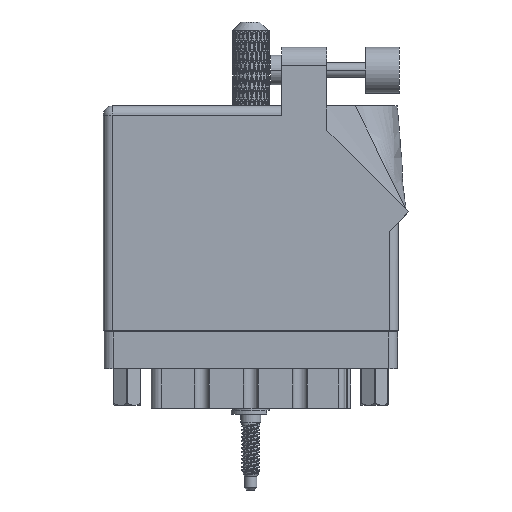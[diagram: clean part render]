
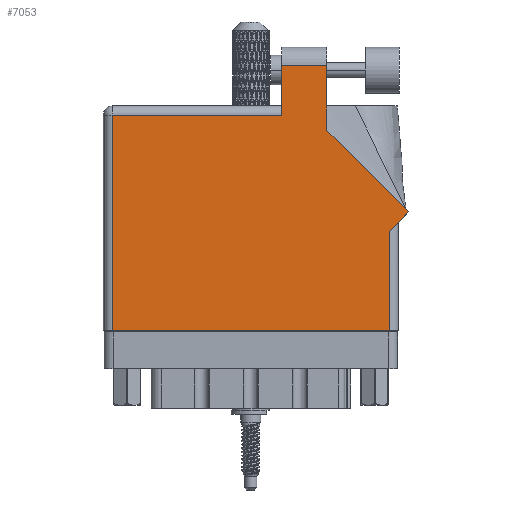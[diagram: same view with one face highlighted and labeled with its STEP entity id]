
A CAD part, front view. The second image highlights one B-rep face of the part: STEP entity #7053.
In plain terms, the highlighted face is planar.
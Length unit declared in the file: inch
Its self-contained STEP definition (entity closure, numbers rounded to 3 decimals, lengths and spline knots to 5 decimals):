
#5122 = VECTOR ( 'NONE', #75772, 39.37008 ) ;
#7053 = ADVANCED_FACE ( 'NONE', ( #70949 ), #7732, .F. ) ;
#7732 = PLANE ( 'NONE',  #76539 ) ;
#9348 = VERTEX_POINT ( 'NONE', #70946 ) ;
#9827 = EDGE_CURVE ( 'NONE', #87743, #76455, #40275, .T. ) ;
#10500 = VERTEX_POINT ( 'NONE', #101364 ) ;
#10588 = LINE ( 'NONE', #63871, #114702 ) ;
#10964 = DIRECTION ( 'NONE',  ( -0.707, 0.707, 0. ) ) ;
#11872 = CARTESIAN_POINT ( 'NONE',  ( 0., 0., 0. ) ) ;
#19192 = CARTESIAN_POINT ( 'NONE',  ( 2.08071, 0.80771, 0. ) ) ;
#19489 = LINE ( 'NONE', #11872, #102658 ) ;
#20319 = LINE ( 'NONE', #19192, #86855 ) ;
#21005 = EDGE_CURVE ( 'NONE', #69353, #87743, #53321, .T. ) ;
#24170 = DIRECTION ( 'NONE',  ( 0., 1., 0. ) ) ;
#26966 = CARTESIAN_POINT ( 'NONE',  ( 1.217, 1.53, 0. ) ) ;
#28724 = CARTESIAN_POINT ( 'NONE',  ( 0.062, 0., 0. ) ) ;
#29617 = CARTESIAN_POINT ( 'NONE',  ( 1.524, 1.36442, 0. ) ) ;
#31283 = ORIENTED_EDGE ( 'NONE', *, *, #49875, .T. ) ;
#36692 = CARTESIAN_POINT ( 'NONE',  ( 1.948, 0.675, 0. ) ) ;
#36913 = EDGE_CURVE ( 'NONE', #74993, #54973, #49385, .T. ) ;
#40275 = LINE ( 'NONE', #84242, #65567 ) ;
#45832 = DIRECTION ( 'NONE',  ( 1., 0., 0. ) ) ;
#45952 = CARTESIAN_POINT ( 'NONE',  ( 1.217, 1.805, 0. ) ) ;
#46294 = DIRECTION ( 'NONE',  ( -1., 0., 0. ) ) ;
#48882 = ORIENTED_EDGE ( 'NONE', *, *, #9827, .T. ) ;
#49385 = LINE ( 'NONE', #74615, #5122 ) ;
#49875 = EDGE_CURVE ( 'NONE', #76455, #114369, #55099, .T. ) ;
#52419 = VERTEX_POINT ( 'NONE', #78527 ) ;
#53061 = EDGE_CURVE ( 'NONE', #114369, #52419, #19489, .T. ) ;
#53321 = LINE ( 'NONE', #26966, #95538 ) ;
#53946 = DIRECTION ( 'NONE',  ( 0., 0., -1. ) ) ;
#54632 = ORIENTED_EDGE ( 'NONE', *, *, #82011, .T. ) ;
#54973 = VERTEX_POINT ( 'NONE', #89407 ) ;
#55099 = LINE ( 'NONE', #28724, #55949 ) ;
#55949 = VECTOR ( 'NONE', #88098, 39.37008 ) ;
#63018 = DIRECTION ( 'NONE',  ( 0., 1., 0. ) ) ;
#63837 = CARTESIAN_POINT ( 'NONE',  ( 1.217, 1.468, 0. ) ) ;
#63871 = CARTESIAN_POINT ( 'NONE',  ( 1.217, 1.805, 0. ) ) ;
#65360 = VECTOR ( 'NONE', #24170, 39.37008 ) ;
#65567 = VECTOR ( 'NONE', #83099, 39.37008 ) ;
#68652 = LINE ( 'NONE', #111467, #65360 ) ;
#69353 = VERTEX_POINT ( 'NONE', #45952 ) ;
#69464 = ORIENTED_EDGE ( 'NONE', *, *, #90714, .T. ) ;
#70946 = CARTESIAN_POINT ( 'NONE',  ( 1.524, 1.805, 0. ) ) ;
#70949 = FACE_OUTER_BOUND ( 'NONE', #88864, .T. ) ;
#72392 = ORIENTED_EDGE ( 'NONE', *, *, #53061, .T. ) ;
#74615 = CARTESIAN_POINT ( 'NONE',  ( 2.01, 0.737, 0. ) ) ;
#74993 = VERTEX_POINT ( 'NONE', #36692 ) ;
#75772 = DIRECTION ( 'NONE',  ( 0.707, 0.707, 0. ) ) ;
#76455 = VERTEX_POINT ( 'NONE', #80378 ) ;
#76539 = AXIS2_PLACEMENT_3D ( 'NONE', #89716, #53946, #106692 ) ;
#77717 = VECTOR ( 'NONE', #63018, 39.37008 ) ;
#78527 = CARTESIAN_POINT ( 'NONE',  ( 1.948, 0., 0. ) ) ;
#80378 = CARTESIAN_POINT ( 'NONE',  ( 0.062, 1.468, 0. ) ) ;
#82011 = EDGE_CURVE ( 'NONE', #52419, #74993, #68652, .T. ) ;
#83099 = DIRECTION ( 'NONE',  ( -1., 0., 0. ) ) ;
#84242 = CARTESIAN_POINT ( 'NONE',  ( 0., 1.468, 0. ) ) ;
#84872 = ORIENTED_EDGE ( 'NONE', *, *, #97023, .T. ) ;
#86855 = VECTOR ( 'NONE', #10964, 39.37008 ) ;
#87743 = VERTEX_POINT ( 'NONE', #63837 ) ;
#88098 = DIRECTION ( 'NONE',  ( 0., -1., 0. ) ) ;
#88864 = EDGE_LOOP ( 'NONE', ( #114914, #69464, #114486, #48882, #31283, #72392, #54632, #109570, #84872 ) ) ;
#89407 = CARTESIAN_POINT ( 'NONE',  ( 2.08071, 0.80771, 0. ) ) ;
#89665 = DIRECTION ( 'NONE',  ( 0., -1., 0. ) ) ;
#89716 = CARTESIAN_POINT ( 'NONE',  ( 0., 1.53, 0. ) ) ;
#90714 = EDGE_CURVE ( 'NONE', #9348, #69353, #10588, .T. ) ;
#95538 = VECTOR ( 'NONE', #89665, 39.37008 ) ;
#97023 = EDGE_CURVE ( 'NONE', #54973, #10500, #20319, .T. ) ;
#99343 = LINE ( 'NONE', #29617, #77717 ) ;
#101364 = CARTESIAN_POINT ( 'NONE',  ( 1.524, 1.36442, 0. ) ) ;
#102658 = VECTOR ( 'NONE', #45832, 39.37008 ) ;
#106692 = DIRECTION ( 'NONE',  ( -1., 0., 0. ) ) ;
#106904 = EDGE_CURVE ( 'NONE', #10500, #9348, #99343, .T. ) ;
#108501 = CARTESIAN_POINT ( 'NONE',  ( 0.062, 0., 0. ) ) ;
#109570 = ORIENTED_EDGE ( 'NONE', *, *, #36913, .T. ) ;
#111467 = CARTESIAN_POINT ( 'NONE',  ( 1.948, 0.737, 0. ) ) ;
#114369 = VERTEX_POINT ( 'NONE', #108501 ) ;
#114486 = ORIENTED_EDGE ( 'NONE', *, *, #21005, .T. ) ;
#114702 = VECTOR ( 'NONE', #46294, 39.37008 ) ;
#114914 = ORIENTED_EDGE ( 'NONE', *, *, #106904, .T. ) ;
